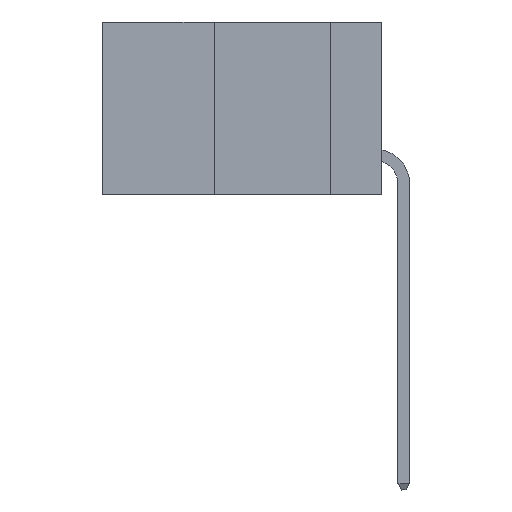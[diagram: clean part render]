
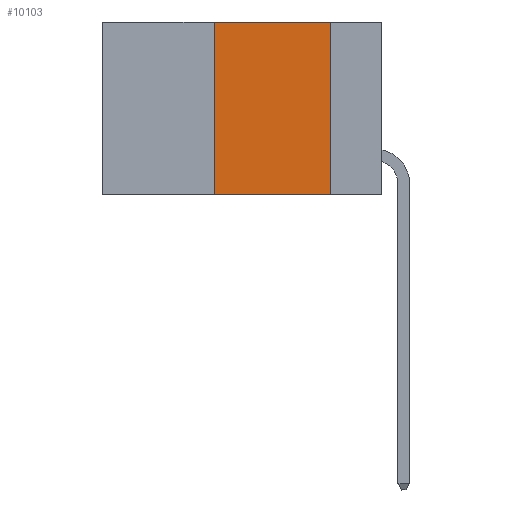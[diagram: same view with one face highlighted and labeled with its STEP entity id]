
A CAD part, left-side view. The second image highlights one B-rep face of the part: STEP entity #10103.
In plain terms, the highlighted planar face has unit normal (-1, 0, 0).
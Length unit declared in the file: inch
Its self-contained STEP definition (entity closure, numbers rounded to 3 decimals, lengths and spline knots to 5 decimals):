
#51 = ORIENTED_EDGE ( 'NONE', *, *, #2507, .F. ) ;
#67 = FACE_OUTER_BOUND ( 'NONE', #23098, .T. ) ;
#807 = VECTOR ( 'NONE', #10836, 39.37008 ) ;
#2337 = PLANE ( 'NONE',  #11997 ) ;
#2507 = EDGE_CURVE ( 'NONE', #20539, #21780, #25013, .T. ) ;
#3845 = VERTEX_POINT ( 'NONE', #16938 ) ;
#4502 = CARTESIAN_POINT ( 'NONE',  ( 0., 0.36, 0. ) ) ;
#5882 = DIRECTION ( 'NONE',  ( 0., -1., 0. ) ) ;
#7603 = CARTESIAN_POINT ( 'NONE',  ( 0., 0.11, 0. ) ) ;
#10088 = LINE ( 'NONE', #18212, #21808 ) ;
#10103 = ADVANCED_FACE ( 'NONE', ( #67 ), #2337, .F. ) ;
#10836 = DIRECTION ( 'NONE',  ( 0., 0., -1. ) ) ;
#11582 = ORIENTED_EDGE ( 'NONE', *, *, #17460, .F. ) ;
#11800 = VECTOR ( 'NONE', #18856, 39.37008 ) ;
#11997 = AXIS2_PLACEMENT_3D ( 'NONE', #16399, #24624, #20990 ) ;
#13806 = CARTESIAN_POINT ( 'NONE',  ( 0., 0.6, -0.37 ) ) ;
#13931 = DIRECTION ( 'NONE',  ( 0., -1., 0. ) ) ;
#15163 = VECTOR ( 'NONE', #13931, 39.37008 ) ;
#15918 = ORIENTED_EDGE ( 'NONE', *, *, #22699, .T. ) ;
#16243 = ORIENTED_EDGE ( 'NONE', *, *, #24811, .F. ) ;
#16399 = CARTESIAN_POINT ( 'NONE',  ( 0., 0.6, 0. ) ) ;
#16815 = LINE ( 'NONE', #4502, #11800 ) ;
#16919 = CARTESIAN_POINT ( 'NONE',  ( 0., 0.11, 0. ) ) ;
#16938 = CARTESIAN_POINT ( 'NONE',  ( 0., 0.36, 0. ) ) ;
#17460 = EDGE_CURVE ( 'NONE', #22248, #3845, #16815, .T. ) ;
#18212 = CARTESIAN_POINT ( 'NONE',  ( 0., 0.6, 0. ) ) ;
#18856 = DIRECTION ( 'NONE',  ( 0., 0., 1. ) ) ;
#19755 = LINE ( 'NONE', #13806, #15163 ) ;
#20052 = CARTESIAN_POINT ( 'NONE',  ( 0., 0.36, -0.37 ) ) ;
#20539 = VERTEX_POINT ( 'NONE', #7603 ) ;
#20990 = DIRECTION ( 'NONE',  ( 0., 0., -1. ) ) ;
#21780 = VERTEX_POINT ( 'NONE', #24211 ) ;
#21808 = VECTOR ( 'NONE', #5882, 39.37008 ) ;
#22248 = VERTEX_POINT ( 'NONE', #20052 ) ;
#22699 = EDGE_CURVE ( 'NONE', #22248, #21780, #19755, .T. ) ;
#23098 = EDGE_LOOP ( 'NONE', ( #51, #16243, #11582, #15918 ) ) ;
#24211 = CARTESIAN_POINT ( 'NONE',  ( 0., 0.11, -0.37 ) ) ;
#24624 = DIRECTION ( 'NONE',  ( 1., 0., 0. ) ) ;
#24811 = EDGE_CURVE ( 'NONE', #3845, #20539, #10088, .T. ) ;
#25013 = LINE ( 'NONE', #16919, #807 ) ;
